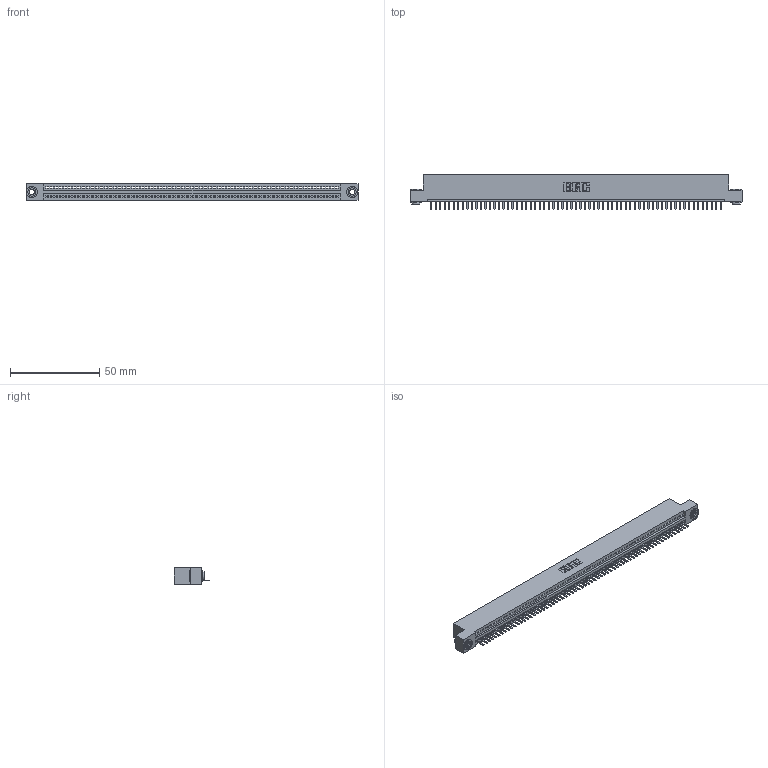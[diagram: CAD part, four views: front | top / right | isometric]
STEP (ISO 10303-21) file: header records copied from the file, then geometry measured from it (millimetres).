
FILE_DESCRIPTION (( 'STEP AP203' ), '1' );
FILE_NAME ('395-065-520-103.STEP', '2019-10-25T03:49:32', ( '' ), ( '' ), 'SwSTEP 2.0', 'SolidWorks 2016', '' );
FILE_SCHEMA (( 'CONFIG_CONTROL_DESIGN' ));
Length unit declared in the file: inch
Products named in the file (4): 345 Part_Flush Mounting Lugs - 0.156 Dia-TH; 345-292-001_345-293-120; 395-065-520-103; 345-250-002_345-250-002-102
Assembly tree (68 placements, depth 2):
  395-065-520-103
    345 Part_Flush Mounting Lugs - 0.156 Dia-TH
    345-292-001_345-293-120  x65
    345-250-002_345-250-002-102  x2
Bounding box: 186.31 x 19.68 x 9.4 mm (x, y, z)
Volume: 17716.6 mm3; surface area: 23459.2 mm2
Topology: 68 solids, 68 shells, 4194 faces, 12377 edges, 8074 vertices
Faces by surface type: plane 2820, cylinder 1366, cone 8
Entity records: 46588 total; most frequent: CARTESIAN_POINT 8058, ORIENTED_EDGE 8038, DIRECTION 7023, EDGE_CURVE 4019, VECTOR 3599, LINE 3599, VERTEX_POINT 2674, AXIS2_PLACEMENT_3D 1712
